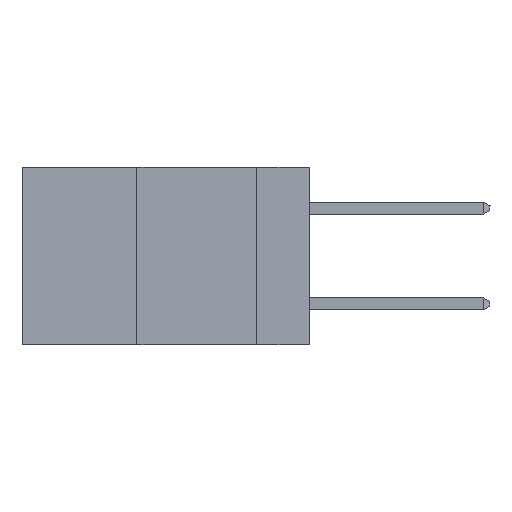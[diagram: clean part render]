
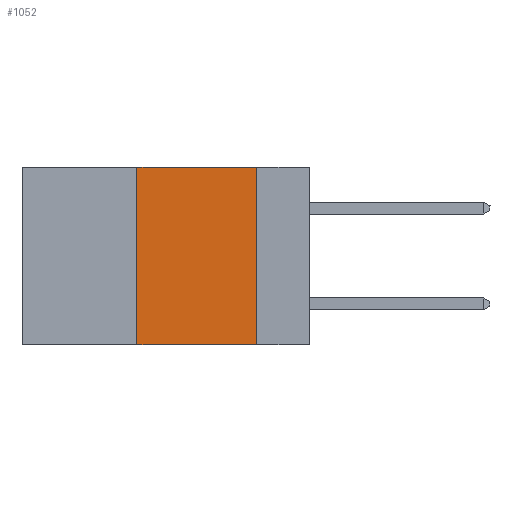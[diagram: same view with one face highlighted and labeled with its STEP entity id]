
A CAD part, left-side view. The second image highlights one B-rep face of the part: STEP entity #1052.
In plain terms, the highlighted planar face has unit normal (-1, 0, 0).
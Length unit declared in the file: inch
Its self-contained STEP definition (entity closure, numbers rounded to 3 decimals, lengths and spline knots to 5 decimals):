
#857 = EDGE_CURVE ( 'NONE', #4694, #14353, #13388, .T. ) ;
#1052 = ADVANCED_FACE ( 'NONE', ( #22357 ), #33265, .F. ) ;
#4694 = VERTEX_POINT ( 'NONE', #14852 ) ;
#6309 = EDGE_LOOP ( 'NONE', ( #27434, #7013, #9994, #16616 ) ) ;
#6491 = VECTOR ( 'NONE', #10775, 39.37008 ) ;
#6765 = DIRECTION ( 'NONE',  ( 0., 0., -1. ) ) ;
#7013 = ORIENTED_EDGE ( 'NONE', *, *, #8018, .F. ) ;
#7145 = DIRECTION ( 'NONE',  ( 0., -1., 0. ) ) ;
#7239 = AXIS2_PLACEMENT_3D ( 'NONE', #12150, #9714, #6765 ) ;
#7933 = VECTOR ( 'NONE', #14107, 39.37008 ) ;
#8018 = EDGE_CURVE ( 'NONE', #14353, #22595, #22736, .T. ) ;
#9714 = DIRECTION ( 'NONE',  ( 1., 0., 0. ) ) ;
#9994 = ORIENTED_EDGE ( 'NONE', *, *, #857, .F. ) ;
#10775 = DIRECTION ( 'NONE',  ( 0., 0., 1. ) ) ;
#12150 = CARTESIAN_POINT ( 'NONE',  ( 0., 0.6, 0. ) ) ;
#12524 = DIRECTION ( 'NONE',  ( 0., -1., 0. ) ) ;
#13388 = LINE ( 'NONE', #15810, #6491 ) ;
#14107 = DIRECTION ( 'NONE',  ( 0., 0., -1. ) ) ;
#14353 = VERTEX_POINT ( 'NONE', #33028 ) ;
#14742 = VECTOR ( 'NONE', #7145, 39.37008 ) ;
#14852 = CARTESIAN_POINT ( 'NONE',  ( 0., 0.36, -0.37 ) ) ;
#15161 = EDGE_CURVE ( 'NONE', #22595, #15366, #27254, .T. ) ;
#15366 = VERTEX_POINT ( 'NONE', #21638 ) ;
#15810 = CARTESIAN_POINT ( 'NONE',  ( 0., 0.36, 0. ) ) ;
#16616 = ORIENTED_EDGE ( 'NONE', *, *, #25166, .T. ) ;
#18071 = CARTESIAN_POINT ( 'NONE',  ( 0., 0.6, -0.37 ) ) ;
#20159 = LINE ( 'NONE', #18071, #14742 ) ;
#21551 = CARTESIAN_POINT ( 'NONE',  ( 0., 0.11, 0. ) ) ;
#21638 = CARTESIAN_POINT ( 'NONE',  ( 0., 0.11, -0.37 ) ) ;
#22357 = FACE_OUTER_BOUND ( 'NONE', #6309, .T. ) ;
#22595 = VERTEX_POINT ( 'NONE', #32266 ) ;
#22624 = VECTOR ( 'NONE', #12524, 39.37008 ) ;
#22736 = LINE ( 'NONE', #23246, #22624 ) ;
#23246 = CARTESIAN_POINT ( 'NONE',  ( 0., 0.6, 0. ) ) ;
#25166 = EDGE_CURVE ( 'NONE', #4694, #15366, #20159, .T. ) ;
#27254 = LINE ( 'NONE', #21551, #7933 ) ;
#27434 = ORIENTED_EDGE ( 'NONE', *, *, #15161, .F. ) ;
#32266 = CARTESIAN_POINT ( 'NONE',  ( 0., 0.11, 0. ) ) ;
#33028 = CARTESIAN_POINT ( 'NONE',  ( 0., 0.36, 0. ) ) ;
#33265 = PLANE ( 'NONE',  #7239 ) ;
